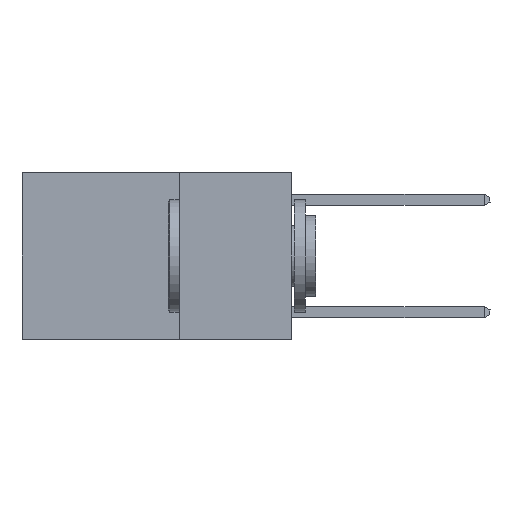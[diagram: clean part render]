
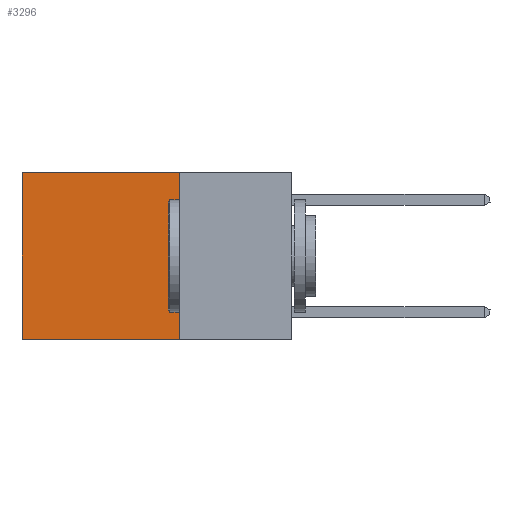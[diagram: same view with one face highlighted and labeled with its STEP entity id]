
A CAD part, left-side view. The second image highlights one B-rep face of the part: STEP entity #3296.
In plain terms, the highlighted planar face has unit normal (-1, 0, 0).
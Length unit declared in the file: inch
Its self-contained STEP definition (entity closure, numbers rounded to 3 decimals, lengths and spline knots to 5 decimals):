
#177 = DIRECTION ( 'NONE',  ( 0., 1., 0. ) ) ;
#425 = ORIENTED_EDGE ( 'NONE', *, *, #4774, .F. ) ;
#1063 = PLANE ( 'NONE',  #12154 ) ;
#1075 = VERTEX_POINT ( 'NONE', #11631 ) ;
#1776 = VERTEX_POINT ( 'NONE', #11393 ) ;
#2311 = CARTESIAN_POINT ( 'NONE',  ( 0.2625, 0.6, -0.37 ) ) ;
#2456 = FACE_OUTER_BOUND ( 'NONE', #4724, .T. ) ;
#3142 = ORIENTED_EDGE ( 'NONE', *, *, #5922, .F. ) ;
#3296 = ADVANCED_FACE ( 'NONE', ( #2456 ), #1063, .F. ) ;
#4410 = VERTEX_POINT ( 'NONE', #10347 ) ;
#4724 = EDGE_LOOP ( 'NONE', ( #5814, #425, #3142, #4924 ) ) ;
#4774 = EDGE_CURVE ( 'NONE', #1776, #9007, #10019, .T. ) ;
#4797 = DIRECTION ( 'NONE',  ( 1., 0., 0. ) ) ;
#4924 = ORIENTED_EDGE ( 'NONE', *, *, #6828, .T. ) ;
#5107 = CARTESIAN_POINT ( 'NONE',  ( 0.2625, 0.25, 0. ) ) ;
#5452 = LINE ( 'NONE', #5107, #8806 ) ;
#5550 = CARTESIAN_POINT ( 'NONE',  ( 0.2625, 0.25, -0.37 ) ) ;
#5621 = DIRECTION ( 'NONE',  ( 0., 1., 0. ) ) ;
#5767 = VECTOR ( 'NONE', #177, 39.37008 ) ;
#5814 = ORIENTED_EDGE ( 'NONE', *, *, #6227, .T. ) ;
#5851 = DIRECTION ( 'NONE',  ( 0., 0., -1. ) ) ;
#5922 = EDGE_CURVE ( 'NONE', #4410, #1776, #5452, .T. ) ;
#6042 = CARTESIAN_POINT ( 'NONE',  ( 0.2625, 0.25, 0. ) ) ;
#6227 = EDGE_CURVE ( 'NONE', #1075, #9007, #10746, .T. ) ;
#6828 = EDGE_CURVE ( 'NONE', #4410, #1075, #11378, .T. ) ;
#7018 = DIRECTION ( 'NONE',  ( 0., 0., -1. ) ) ;
#7790 = CARTESIAN_POINT ( 'NONE',  ( 0.2625, 0.25, 0. ) ) ;
#8326 = VECTOR ( 'NONE', #5851, 39.37008 ) ;
#8806 = VECTOR ( 'NONE', #7018, 39.37008 ) ;
#9007 = VERTEX_POINT ( 'NONE', #2311 ) ;
#9839 = CARTESIAN_POINT ( 'NONE',  ( 0.2625, 0.6, 0. ) ) ;
#10019 = LINE ( 'NONE', #5550, #10035 ) ;
#10035 = VECTOR ( 'NONE', #5621, 39.37008 ) ;
#10347 = CARTESIAN_POINT ( 'NONE',  ( 0.2625, 0.25, 0. ) ) ;
#10682 = DIRECTION ( 'NONE',  ( 0., 0., -1. ) ) ;
#10746 = LINE ( 'NONE', #9839, #8326 ) ;
#11378 = LINE ( 'NONE', #6042, #5767 ) ;
#11393 = CARTESIAN_POINT ( 'NONE',  ( 0.2625, 0.25, -0.37 ) ) ;
#11631 = CARTESIAN_POINT ( 'NONE',  ( 0.2625, 0.6, 0. ) ) ;
#12154 = AXIS2_PLACEMENT_3D ( 'NONE', #7790, #4797, #10682 ) ;
